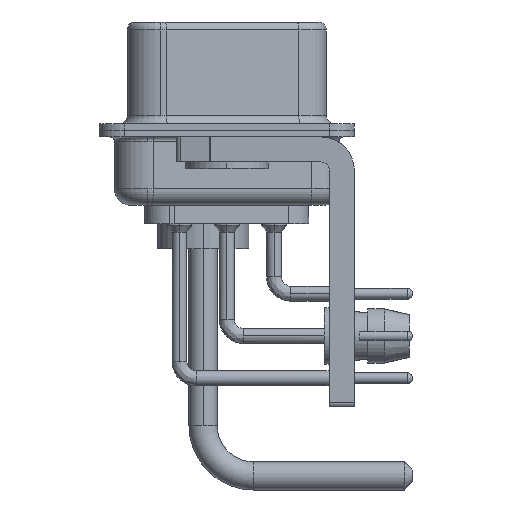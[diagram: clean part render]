
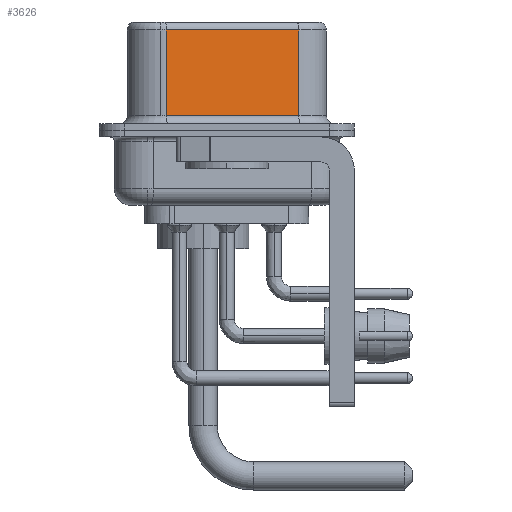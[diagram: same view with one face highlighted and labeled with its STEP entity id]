
A CAD part, left-side view. The second image highlights one B-rep face of the part: STEP entity #3626.
In plain terms, the highlighted planar face has unit normal (-0.985, -0.174, 0).
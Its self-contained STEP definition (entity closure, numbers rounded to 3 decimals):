
#1558 = ORIENTED_EDGE ( 'NONE', *, *, #17744, .T. ) ;
#1911 = AXIS2_PLACEMENT_3D ( 'NONE', #22183, #15753, #16556 ) ;
#2472 = DIRECTION ( 'NONE',  ( 0., 0., -1. ) ) ;
#2891 = ORIENTED_EDGE ( 'NONE', *, *, #35678, .T. ) ;
#3626 = ADVANCED_FACE ( 'NONE', ( #28846 ), #34650, .F. ) ;
#4814 = VECTOR ( 'NONE', #37045, 1000. ) ;
#4951 = DIRECTION ( 'NONE',  ( 0.174, -0.985, 0. ) ) ;
#5279 = LINE ( 'NONE', #17564, #21783 ) ;
#9539 = VERTEX_POINT ( 'NONE', #14038 ) ;
#10974 = VERTEX_POINT ( 'NONE', #30517 ) ;
#14016 = VECTOR ( 'NONE', #4951, 1000. ) ;
#14038 = CARTESIAN_POINT ( 'NONE',  ( 5.132, -4.322, 6.02 ) ) ;
#15728 = CARTESIAN_POINT ( 'NONE',  ( 5.132, -4.322, 0.9 ) ) ;
#15753 = DIRECTION ( 'NONE',  ( 0.985, 0.174, 0. ) ) ;
#16556 = DIRECTION ( 'NONE',  ( -0.174, 0.985, 0. ) ) ;
#16855 = LINE ( 'NONE', #26696, #14016 ) ;
#17564 = CARTESIAN_POINT ( 'NONE',  ( 5.132, -4.322, 6.52 ) ) ;
#17744 = EDGE_CURVE ( 'NONE', #10974, #21233, #26488, .T. ) ;
#18168 = CARTESIAN_POINT ( 'NONE',  ( 5.132, -4.322, 6.02 ) ) ;
#18350 = LINE ( 'NONE', #18168, #4814 ) ;
#18772 = EDGE_LOOP ( 'NONE', ( #30508, #29595, #1558, #2891 ) ) ;
#21233 = VERTEX_POINT ( 'NONE', #25458 ) ;
#21783 = VECTOR ( 'NONE', #2472, 1000. ) ;
#22183 = CARTESIAN_POINT ( 'NONE',  ( 5.132, -4.322, 6.52 ) ) ;
#22639 = VECTOR ( 'NONE', #35520, 1000. ) ;
#25458 = CARTESIAN_POINT ( 'NONE',  ( 3.73, 3.628, 0.9 ) ) ;
#25895 = CARTESIAN_POINT ( 'NONE',  ( 3.73, 3.628, 6.52 ) ) ;
#26488 = LINE ( 'NONE', #25895, #22639 ) ;
#26696 = CARTESIAN_POINT ( 'NONE',  ( 5.132, -4.322, 0.9 ) ) ;
#28846 = FACE_OUTER_BOUND ( 'NONE', #18772, .T. ) ;
#29595 = ORIENTED_EDGE ( 'NONE', *, *, #33260, .T. ) ;
#30508 = ORIENTED_EDGE ( 'NONE', *, *, #36905, .F. ) ;
#30517 = CARTESIAN_POINT ( 'NONE',  ( 3.73, 3.628, 6.02 ) ) ;
#33260 = EDGE_CURVE ( 'NONE', #9539, #10974, #18350, .T. ) ;
#34524 = VERTEX_POINT ( 'NONE', #15728 ) ;
#34650 = PLANE ( 'NONE',  #1911 ) ;
#35520 = DIRECTION ( 'NONE',  ( 0., 0., -1. ) ) ;
#35678 = EDGE_CURVE ( 'NONE', #21233, #34524, #16855, .T. ) ;
#36905 = EDGE_CURVE ( 'NONE', #9539, #34524, #5279, .T. ) ;
#37045 = DIRECTION ( 'NONE',  ( -0.174, 0.985, 0. ) ) ;
